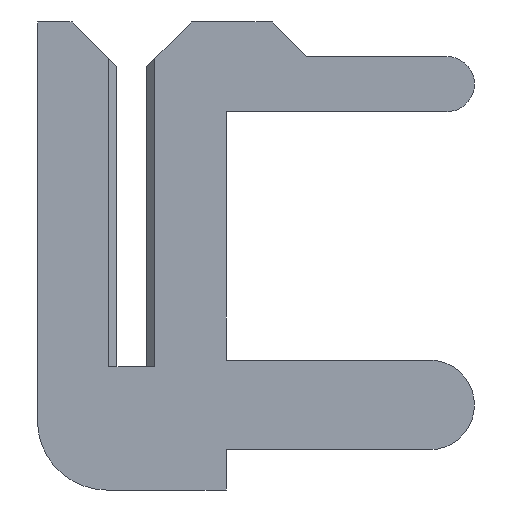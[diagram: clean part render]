
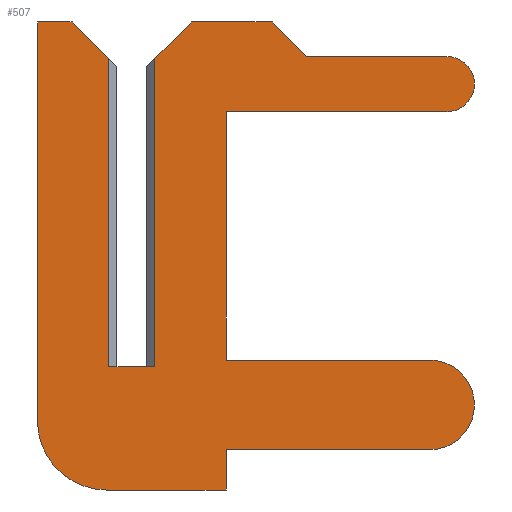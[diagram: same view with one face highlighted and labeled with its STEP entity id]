
A CAD part, left-side view. The second image highlights one B-rep face of the part: STEP entity #507.
In plain terms, the highlighted planar face has unit normal (-1, 0, 0).
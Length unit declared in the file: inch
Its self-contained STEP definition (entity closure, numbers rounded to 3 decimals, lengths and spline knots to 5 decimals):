
#1 = LINE ( 'NONE', #135, #420 ) ;
#3 = EDGE_CURVE ( 'NONE', #447, #979, #572, .T. ) ;
#6 = CARTESIAN_POINT ( 'NONE',  ( -0.01, 0.01, -0.0235 ) ) ;
#10 = EDGE_CURVE ( 'NONE', #252, #1117, #724, .T. ) ;
#26 = ORIENTED_EDGE ( 'NONE', *, *, #104, .F. ) ;
#27 = ORIENTED_EDGE ( 'NONE', *, *, #525, .F. ) ;
#30 = LINE ( 'NONE', #1049, #814 ) ;
#44 = ORIENTED_EDGE ( 'NONE', *, *, #283, .F. ) ;
#48 = DIRECTION ( 'NONE',  ( 0., 0., -1. ) ) ;
#65 = EDGE_CURVE ( 'NONE', #696, #653, #785, .T. ) ;
#82 = DIRECTION ( 'NONE',  ( 0., 0., 1. ) ) ;
#95 = CARTESIAN_POINT ( 'NONE',  ( -0.01, -0.041, -0.0535 ) ) ;
#100 = CARTESIAN_POINT ( 'NONE',  ( -0.01, -0.041, -0.0535 ) ) ;
#104 = EDGE_CURVE ( 'NONE', #464, #829, #1, .T. ) ;
#106 = DIRECTION ( 'NONE',  ( 0., 1., 0. ) ) ;
#107 = DIRECTION ( 'NONE',  ( 0., -1., 0. ) ) ;
#123 = CARTESIAN_POINT ( 'NONE',  ( -0.01, -0.137, 0.123 ) ) ;
#125 = ORIENTED_EDGE ( 'NONE', *, *, #428, .F. ) ;
#135 = CARTESIAN_POINT ( 'NONE',  ( -0.01, -0.137, 0.135 ) ) ;
#170 = VECTOR ( 'NONE', #1101, 39.37008 ) ;
#179 = CARTESIAN_POINT ( 'NONE',  ( -0.01, -0.1295, 0.003 ) ) ;
#184 = CARTESIAN_POINT ( 'NONE',  ( -0.01, 0.026, 0.15 ) ) ;
#199 = EDGE_CURVE ( 'NONE', #1052, #1016, #1017, .T. ) ;
#202 = ORIENTED_EDGE ( 'NONE', *, *, #398, .F. ) ;
#205 = VECTOR ( 'NONE', #261, 39.37008 ) ;
#217 = VERTEX_POINT ( 'NONE', #1137 ) ;
#239 = FACE_OUTER_BOUND ( 'NONE', #528, .T. ) ;
#252 = VERTEX_POINT ( 'NONE', #256 ) ;
#254 = ORIENTED_EDGE ( 'NONE', *, *, #963, .F. ) ;
#256 = CARTESIAN_POINT ( 'NONE',  ( -0.01, 0.011, -0.0535 ) ) ;
#258 = CARTESIAN_POINT ( 'NONE',  ( -0.01, -0.076, 0.135 ) ) ;
#261 = DIRECTION ( 'NONE',  ( 0., -0.707, -0.707 ) ) ;
#269 = DIRECTION ( 'NONE',  ( 0., -0.707, -0.707 ) ) ;
#273 = DIRECTION ( 'NONE',  ( 0., -1., 0. ) ) ;
#283 = EDGE_CURVE ( 'NONE', #979, #414, #319, .T. ) ;
#286 = VECTOR ( 'NONE', #269, 39.37008 ) ;
#300 = CARTESIAN_POINT ( 'NONE',  ( -0.01, -0.076, 0.135 ) ) ;
#302 = VERTEX_POINT ( 'NONE', #323 ) ;
#309 = VECTOR ( 'NONE', #459, 39.37008 ) ;
#319 = LINE ( 'NONE', #862, #531 ) ;
#320 = VECTOR ( 'NONE', #354, 39.37008 ) ;
#323 = CARTESIAN_POINT ( 'NONE',  ( -0.01, -0.026, 0.15 ) ) ;
#333 = ORIENTED_EDGE ( 'NONE', *, *, #931, .F. ) ;
#334 = ORIENTED_EDGE ( 'NONE', *, *, #1013, .F. ) ;
#337 = VECTOR ( 'NONE', #106, 39.37008 ) ;
#340 = VECTOR ( 'NONE', #273, 39.37008 ) ;
#342 = EDGE_CURVE ( 'NONE', #839, #252, #30, .T. ) ;
#352 = CARTESIAN_POINT ( 'NONE',  ( -0.01, 0.041, 0.15 ) ) ;
#353 = LINE ( 'NONE', #100, #309 ) ;
#354 = DIRECTION ( 'NONE',  ( 0., 0., 1. ) ) ;
#355 = AXIS2_PLACEMENT_3D ( 'NONE', #361, #538, #885 ) ;
#356 = DIRECTION ( 'NONE',  ( 0., -1., 0. ) ) ;
#359 = CARTESIAN_POINT ( 'NONE',  ( -0.01, -0.1295, 0.003 ) ) ;
#361 = CARTESIAN_POINT ( 'NONE',  ( -0.01, 0.011, -0.0235 ) ) ;
#373 = CARTESIAN_POINT ( 'NONE',  ( -0.01, -0.1295, -0.036 ) ) ;
#392 = DIRECTION ( 'NONE',  ( 1., 0., 0. ) ) ;
#398 = EDGE_CURVE ( 'NONE', #217, #653, #911, .T. ) ;
#414 = VERTEX_POINT ( 'NONE', #594 ) ;
#420 = VECTOR ( 'NONE', #1030, 39.37008 ) ;
#428 = EDGE_CURVE ( 'NONE', #414, #1054, #655, .T. ) ;
#443 = EDGE_CURVE ( 'NONE', #1117, #981, #714, .T. ) ;
#447 = VERTEX_POINT ( 'NONE', #987 ) ;
#452 = AXIS2_PLACEMENT_3D ( 'NONE', #123, #392, #746 ) ;
#459 = DIRECTION ( 'NONE',  ( 0., 0., -1. ) ) ;
#464 = VERTEX_POINT ( 'NONE', #258 ) ;
#465 = ORIENTED_EDGE ( 'NONE', *, *, #342, .F. ) ;
#478 = CARTESIAN_POINT ( 'NONE',  ( -0.01, -0.061, 0.15 ) ) ;
#482 = CARTESIAN_POINT ( 'NONE',  ( -0.01, -0.1295, -0.0165 ) ) ;
#506 = LINE ( 'NONE', #6, #320 ) ;
#507 = ADVANCED_FACE ( 'NONE', ( #239 ), #618, .T. ) ;
#525 = EDGE_CURVE ( 'NONE', #1036, #1110, #969, .T. ) ;
#528 = EDGE_LOOP ( 'NONE', ( #951, #769, #202, #796, #27, #851, #568, #1155, #465, #334, #623, #333, #125, #44, #656, #672, #26, #254, #882 ) ) ;
#531 = VECTOR ( 'NONE', #691, 39.37008 ) ;
#534 = CARTESIAN_POINT ( 'NONE',  ( -0.01, -0.026, 0.15 ) ) ;
#538 = DIRECTION ( 'NONE',  ( -1., 0., 0. ) ) ;
#568 = ORIENTED_EDGE ( 'NONE', *, *, #443, .F. ) ;
#571 = DIRECTION ( 'NONE',  ( 1., 0., 0. ) ) ;
#572 = LINE ( 'NONE', #717, #337 ) ;
#583 = AXIS2_PLACEMENT_3D ( 'NONE', #816, #732, #915 ) ;
#589 = EDGE_CURVE ( 'NONE', #217, #1110, #506, .T. ) ;
#594 = CARTESIAN_POINT ( 'NONE',  ( -0.01, -0.041, 0.003 ) ) ;
#611 = DIRECTION ( 'NONE',  ( 0., 1., 0. ) ) ;
#618 = PLANE ( 'NONE',  #355 ) ;
#623 = ORIENTED_EDGE ( 'NONE', *, *, #199, .F. ) ;
#625 = CARTESIAN_POINT ( 'NONE',  ( -0.01, 0.01, 0.134 ) ) ;
#632 = CARTESIAN_POINT ( 'NONE',  ( -0.01, 0.041, 0.15 ) ) ;
#638 = CARTESIAN_POINT ( 'NONE',  ( -0.01, -0.041, -0.036 ) ) ;
#653 = VERTEX_POINT ( 'NONE', #827 ) ;
#655 = LINE ( 'NONE', #179, #340 ) ;
#656 = ORIENTED_EDGE ( 'NONE', *, *, #3, .F. ) ;
#672 = ORIENTED_EDGE ( 'NONE', *, *, #907, .F. ) ;
#675 = LINE ( 'NONE', #1095, #170 ) ;
#677 = CARTESIAN_POINT ( 'NONE',  ( -0.01, -0.01, 0.15 ) ) ;
#688 = VECTOR ( 'NONE', #82, 39.37008 ) ;
#691 = DIRECTION ( 'NONE',  ( 0., 0., -1. ) ) ;
#696 = VERTEX_POINT ( 'NONE', #995 ) ;
#704 = VECTOR ( 'NONE', #107, 39.37008 ) ;
#714 = LINE ( 'NONE', #352, #688 ) ;
#716 = CARTESIAN_POINT ( 'NONE',  ( -0.01, 0.041, -0.0235 ) ) ;
#717 = CARTESIAN_POINT ( 'NONE',  ( -0.01, -0.041, 0.111 ) ) ;
#724 = CIRCLE ( 'NONE', #583, 0.03 ) ;
#732 = DIRECTION ( 'NONE',  ( 1., 0., 0. ) ) ;
#740 = DIRECTION ( 'NONE',  ( 0., 0., 1. ) ) ;
#746 = DIRECTION ( 'NONE',  ( 0., 0., 1. ) ) ;
#769 = ORIENTED_EDGE ( 'NONE', *, *, #65, .T. ) ;
#785 = LINE ( 'NONE', #677, #925 ) ;
#796 = ORIENTED_EDGE ( 'NONE', *, *, #589, .T. ) ;
#801 = CARTESIAN_POINT ( 'NONE',  ( -0.01, 0.0065, 0.1305 ) ) ;
#810 = CARTESIAN_POINT ( 'NONE',  ( -0.01, -0.041, 0.111 ) ) ;
#814 = VECTOR ( 'NONE', #611, 39.37008 ) ;
#816 = CARTESIAN_POINT ( 'NONE',  ( -0.01, 0.011, -0.0235 ) ) ;
#827 = CARTESIAN_POINT ( 'NONE',  ( -0.01, -0.01, 0. ) ) ;
#829 = VERTEX_POINT ( 'NONE', #1090 ) ;
#831 = EDGE_CURVE ( 'NONE', #696, #302, #675, .T. ) ;
#839 = VERTEX_POINT ( 'NONE', #95 ) ;
#848 = CARTESIAN_POINT ( 'NONE',  ( -0.01, -0.041, -0.036 ) ) ;
#851 = ORIENTED_EDGE ( 'NONE', *, *, #994, .F. ) ;
#862 = CARTESIAN_POINT ( 'NONE',  ( -0.01, -0.041, 0.003 ) ) ;
#873 = LINE ( 'NONE', #534, #704 ) ;
#882 = ORIENTED_EDGE ( 'NONE', *, *, #986, .F. ) ;
#885 = DIRECTION ( 'NONE',  ( 0., 0., 1. ) ) ;
#891 = VERTEX_POINT ( 'NONE', #478 ) ;
#892 = VECTOR ( 'NONE', #1037, 39.37008 ) ;
#894 = VECTOR ( 'NONE', #1139, 39.37008 ) ;
#897 = CARTESIAN_POINT ( 'NONE',  ( -0.01, 0.026, 0.15 ) ) ;
#907 = EDGE_CURVE ( 'NONE', #829, #447, #1146, .T. ) ;
#911 = LINE ( 'NONE', #1044, #894 ) ;
#915 = DIRECTION ( 'NONE',  ( 0., 0., 1. ) ) ;
#925 = VECTOR ( 'NONE', #48, 39.37008 ) ;
#931 = EDGE_CURVE ( 'NONE', #1054, #1052, #1115, .T. ) ;
#942 = LINE ( 'NONE', #184, #1100 ) ;
#951 = ORIENTED_EDGE ( 'NONE', *, *, #831, .F. ) ;
#963 = EDGE_CURVE ( 'NONE', #891, #464, #1130, .T. ) ;
#969 = LINE ( 'NONE', #801, #205 ) ;
#979 = VERTEX_POINT ( 'NONE', #810 ) ;
#981 = VERTEX_POINT ( 'NONE', #632 ) ;
#986 = EDGE_CURVE ( 'NONE', #302, #891, #873, .T. ) ;
#987 = CARTESIAN_POINT ( 'NONE',  ( -0.01, -0.137, 0.111 ) ) ;
#994 = EDGE_CURVE ( 'NONE', #981, #1036, #942, .T. ) ;
#995 = CARTESIAN_POINT ( 'NONE',  ( -0.01, -0.01, 0.134 ) ) ;
#1013 = EDGE_CURVE ( 'NONE', #1016, #839, #353, .T. ) ;
#1016 = VERTEX_POINT ( 'NONE', #638 ) ;
#1017 = LINE ( 'NONE', #848, #892 ) ;
#1030 = DIRECTION ( 'NONE',  ( 0., -1., 0. ) ) ;
#1036 = VERTEX_POINT ( 'NONE', #897 ) ;
#1037 = DIRECTION ( 'NONE',  ( 0., 1., 0. ) ) ;
#1044 = CARTESIAN_POINT ( 'NONE',  ( -0.01, 0.0065, 0. ) ) ;
#1049 = CARTESIAN_POINT ( 'NONE',  ( -0.01, 0.011, -0.0535 ) ) ;
#1052 = VERTEX_POINT ( 'NONE', #373 ) ;
#1054 = VERTEX_POINT ( 'NONE', #359 ) ;
#1067 = AXIS2_PLACEMENT_3D ( 'NONE', #482, #571, #740 ) ;
#1090 = CARTESIAN_POINT ( 'NONE',  ( -0.01, -0.137, 0.135 ) ) ;
#1095 = CARTESIAN_POINT ( 'NONE',  ( -0.01, -0.0065, 0.1305 ) ) ;
#1100 = VECTOR ( 'NONE', #356, 39.37008 ) ;
#1101 = DIRECTION ( 'NONE',  ( 0., -0.707, 0.707 ) ) ;
#1110 = VERTEX_POINT ( 'NONE', #625 ) ;
#1115 = CIRCLE ( 'NONE', #1067, 0.0195 ) ;
#1117 = VERTEX_POINT ( 'NONE', #716 ) ;
#1130 = LINE ( 'NONE', #300, #286 ) ;
#1137 = CARTESIAN_POINT ( 'NONE',  ( -0.01, 0.01, 0. ) ) ;
#1139 = DIRECTION ( 'NONE',  ( 0., -1., 0. ) ) ;
#1146 = CIRCLE ( 'NONE', #452, 0.012 ) ;
#1155 = ORIENTED_EDGE ( 'NONE', *, *, #10, .F. ) ;
